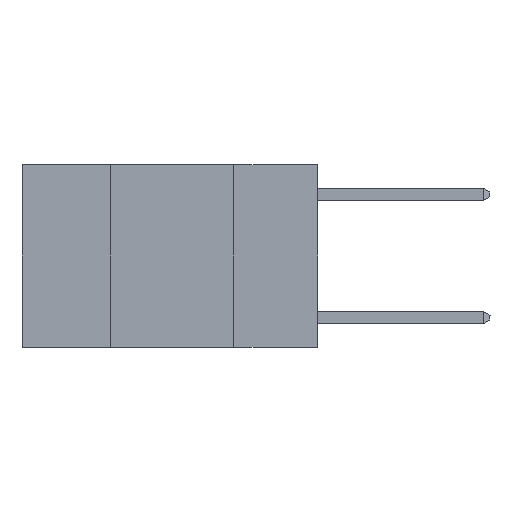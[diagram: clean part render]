
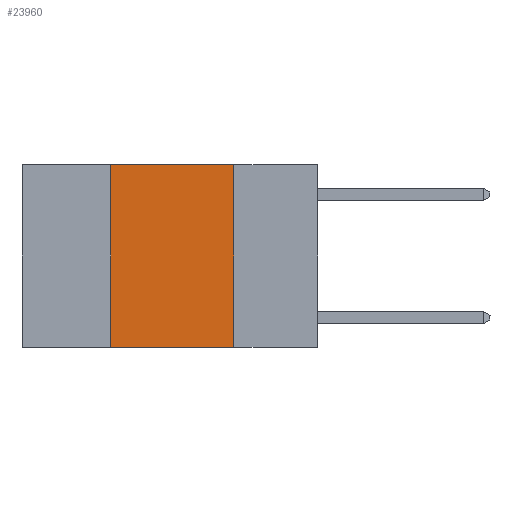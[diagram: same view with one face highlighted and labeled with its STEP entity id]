
A CAD part, left-side view. The second image highlights one B-rep face of the part: STEP entity #23960.
In plain terms, the highlighted planar face has unit normal (-1, 0, 0).
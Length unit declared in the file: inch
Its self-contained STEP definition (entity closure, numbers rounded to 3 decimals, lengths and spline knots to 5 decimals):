
#471 = VECTOR ( 'NONE', #19151, 39.37008 ) ;
#721 = EDGE_LOOP ( 'NONE', ( #13408, #26831, #20326, #19338 ) ) ;
#1776 = LINE ( 'NONE', #3836, #11065 ) ;
#2003 = AXIS2_PLACEMENT_3D ( 'NONE', #4654, #21181, #2465 ) ;
#2305 = VERTEX_POINT ( 'NONE', #14876 ) ;
#2465 = DIRECTION ( 'NONE',  ( 0., 0., -1. ) ) ;
#3440 = VERTEX_POINT ( 'NONE', #18477 ) ;
#3836 = CARTESIAN_POINT ( 'NONE',  ( 0., 0.42, 0. ) ) ;
#4517 = PLANE ( 'NONE',  #2003 ) ;
#4654 = CARTESIAN_POINT ( 'NONE',  ( 0., 0.6, 0. ) ) ;
#5420 = EDGE_CURVE ( 'NONE', #24559, #3440, #1776, .T. ) ;
#5549 = CARTESIAN_POINT ( 'NONE',  ( 0., 0.17, 0. ) ) ;
#6990 = CARTESIAN_POINT ( 'NONE',  ( 0., 0.6, 0. ) ) ;
#7533 = VECTOR ( 'NONE', #26314, 39.37008 ) ;
#8214 = EDGE_CURVE ( 'NONE', #3440, #2305, #10818, .T. ) ;
#8988 = CARTESIAN_POINT ( 'NONE',  ( 0., 0.42, -0.37 ) ) ;
#10533 = DIRECTION ( 'NONE',  ( 0., -1., 0. ) ) ;
#10818 = LINE ( 'NONE', #6990, #471 ) ;
#11065 = VECTOR ( 'NONE', #12172, 39.37008 ) ;
#12172 = DIRECTION ( 'NONE',  ( 0., 0., 1. ) ) ;
#12721 = EDGE_CURVE ( 'NONE', #2305, #15916, #21680, .T. ) ;
#13408 = ORIENTED_EDGE ( 'NONE', *, *, #12721, .F. ) ;
#14876 = CARTESIAN_POINT ( 'NONE',  ( 0., 0.17, 0. ) ) ;
#15044 = LINE ( 'NONE', #23236, #23823 ) ;
#15916 = VERTEX_POINT ( 'NONE', #26951 ) ;
#18477 = CARTESIAN_POINT ( 'NONE',  ( 0., 0.42, 0. ) ) ;
#19151 = DIRECTION ( 'NONE',  ( 0., -1., 0. ) ) ;
#19338 = ORIENTED_EDGE ( 'NONE', *, *, #23911, .T. ) ;
#20326 = ORIENTED_EDGE ( 'NONE', *, *, #5420, .F. ) ;
#21181 = DIRECTION ( 'NONE',  ( 1., 0., 0. ) ) ;
#21680 = LINE ( 'NONE', #5549, #7533 ) ;
#23236 = CARTESIAN_POINT ( 'NONE',  ( 0., 0.6, -0.37 ) ) ;
#23823 = VECTOR ( 'NONE', #10533, 39.37008 ) ;
#23911 = EDGE_CURVE ( 'NONE', #24559, #15916, #15044, .T. ) ;
#23960 = ADVANCED_FACE ( 'NONE', ( #25276 ), #4517, .F. ) ;
#24559 = VERTEX_POINT ( 'NONE', #8988 ) ;
#25276 = FACE_OUTER_BOUND ( 'NONE', #721, .T. ) ;
#26314 = DIRECTION ( 'NONE',  ( 0., 0., -1. ) ) ;
#26831 = ORIENTED_EDGE ( 'NONE', *, *, #8214, .F. ) ;
#26951 = CARTESIAN_POINT ( 'NONE',  ( 0., 0.17, -0.37 ) ) ;
